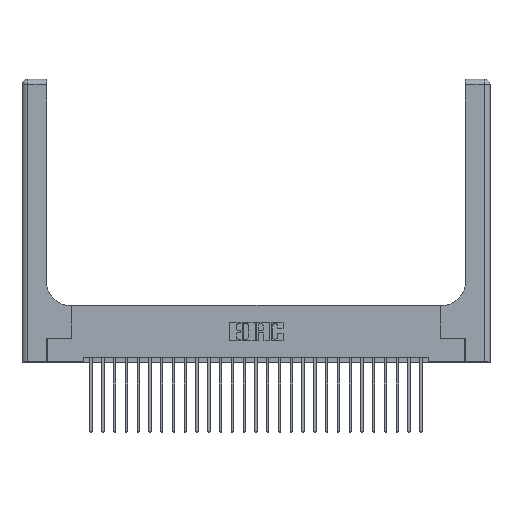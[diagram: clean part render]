
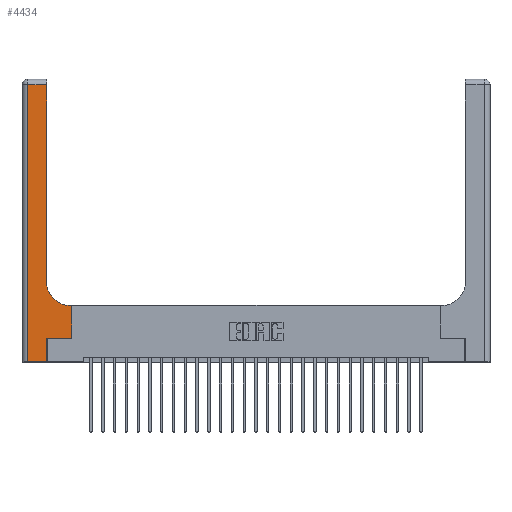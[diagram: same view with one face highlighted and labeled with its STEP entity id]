
A CAD part, top view. The second image highlights one B-rep face of the part: STEP entity #4434.
In plain terms, the highlighted planar face has unit normal (0, 0, 1).
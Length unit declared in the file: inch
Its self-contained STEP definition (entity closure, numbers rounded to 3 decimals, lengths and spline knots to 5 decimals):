
#78 = VERTEX_POINT ( 'NONE', #9043 ) ;
#508 = LINE ( 'NONE', #7594, #12063 ) ;
#548 = LINE ( 'NONE', #16430, #21140 ) ;
#1454 = CARTESIAN_POINT ( 'NONE',  ( 0.528, 0.25, 0.37 ) ) ;
#1733 = ORIENTED_EDGE ( 'NONE', *, *, #17524, .T. ) ;
#2019 = DIRECTION ( 'NONE',  ( -1., 0., 0. ) ) ;
#2164 = CARTESIAN_POINT ( 'NONE',  ( 0.26, 3., 0.37 ) ) ;
#2184 = DIRECTION ( 'NONE',  ( 0., 0., -1. ) ) ;
#2272 = AXIS2_PLACEMENT_3D ( 'NONE', #25510, #25422, #15429 ) ;
#2430 = CARTESIAN_POINT ( 'NONE',  ( 0.528, 0.6, 0.37 ) ) ;
#2673 = VERTEX_POINT ( 'NONE', #6800 ) ;
#2929 = DIRECTION ( 'NONE',  ( 1., 0., 0. ) ) ;
#3951 = DIRECTION ( 'NONE',  ( 0., 1., 0. ) ) ;
#4120 = CARTESIAN_POINT ( 'NONE',  ( 0., 3., 0.37 ) ) ;
#4323 = LINE ( 'NONE', #17794, #13982 ) ;
#4434 = ADVANCED_FACE ( 'NONE', ( #13801 ), #10124, .F. ) ;
#4783 = VERTEX_POINT ( 'NONE', #7234 ) ;
#5087 = CARTESIAN_POINT ( 'NONE',  ( 0.06, 2.94, 0.37 ) ) ;
#5290 = LINE ( 'NONE', #25007, #7183 ) ;
#6087 = CARTESIAN_POINT ( 'NONE',  ( 0.06, 0., 0.37 ) ) ;
#6323 = EDGE_CURVE ( 'NONE', #22401, #2673, #5290, .T. ) ;
#6440 = ORIENTED_EDGE ( 'NONE', *, *, #7628, .T. ) ;
#6583 = VERTEX_POINT ( 'NONE', #2430 ) ;
#6800 = CARTESIAN_POINT ( 'NONE',  ( 0.265, 0., 0.37 ) ) ;
#7183 = VECTOR ( 'NONE', #2929, 39.37008 ) ;
#7234 = CARTESIAN_POINT ( 'NONE',  ( 0.528, 0.25, 0.37 ) ) ;
#7251 = VERTEX_POINT ( 'NONE', #5087 ) ;
#7277 = EDGE_CURVE ( 'NONE', #19356, #11826, #9938, .T. ) ;
#7475 = CARTESIAN_POINT ( 'NONE',  ( 0.51, 0.6, 0.37 ) ) ;
#7594 = CARTESIAN_POINT ( 'NONE',  ( 0.26, 0.6, 0.37 ) ) ;
#7628 = EDGE_CURVE ( 'NONE', #7251, #22401, #548, .T. ) ;
#8007 = CARTESIAN_POINT ( 'NONE',  ( 0.26, 0.85, 0.37 ) ) ;
#8088 = DIRECTION ( 'NONE',  ( -1., 0., 0. ) ) ;
#9043 = CARTESIAN_POINT ( 'NONE',  ( 0.265, 0.25, 0.37 ) ) ;
#9224 = LINE ( 'NONE', #21959, #16116 ) ;
#9255 = EDGE_CURVE ( 'NONE', #6583, #19356, #508, .T. ) ;
#9912 = ORIENTED_EDGE ( 'NONE', *, *, #9255, .T. ) ;
#9938 = CIRCLE ( 'NONE', #2272, 0.25 ) ;
#10124 = PLANE ( 'NONE',  #14109 ) ;
#10501 = DIRECTION ( 'NONE',  ( 0., -1., 0. ) ) ;
#11153 = DIRECTION ( 'NONE',  ( 0., 1., 0. ) ) ;
#11826 = VERTEX_POINT ( 'NONE', #8007 ) ;
#11964 = LINE ( 'NONE', #25677, #25102 ) ;
#12063 = VECTOR ( 'NONE', #21534, 39.37008 ) ;
#13184 = VECTOR ( 'NONE', #15936, 39.37008 ) ;
#13801 = FACE_OUTER_BOUND ( 'NONE', #18793, .T. ) ;
#13982 = VECTOR ( 'NONE', #3951, 39.37008 ) ;
#14109 = AXIS2_PLACEMENT_3D ( 'NONE', #4120, #2184, #2019 ) ;
#14334 = EDGE_CURVE ( 'NONE', #2673, #78, #4323, .T. ) ;
#15190 = EDGE_CURVE ( 'NONE', #4783, #6583, #16409, .T. ) ;
#15260 = DIRECTION ( 'NONE',  ( 1., 0., 0. ) ) ;
#15352 = EDGE_CURVE ( 'NONE', #23142, #7251, #9224, .T. ) ;
#15429 = DIRECTION ( 'NONE',  ( 1., 0., 0. ) ) ;
#15767 = ORIENTED_EDGE ( 'NONE', *, *, #15352, .T. ) ;
#15936 = DIRECTION ( 'NONE',  ( 0., 1., 0. ) ) ;
#16116 = VECTOR ( 'NONE', #8088, 39.37008 ) ;
#16409 = LINE ( 'NONE', #1454, #25185 ) ;
#16430 = CARTESIAN_POINT ( 'NONE',  ( 0.06, 3., 0.37 ) ) ;
#16789 = ORIENTED_EDGE ( 'NONE', *, *, #15190, .T. ) ;
#17359 = ORIENTED_EDGE ( 'NONE', *, *, #23991, .T. ) ;
#17524 = EDGE_CURVE ( 'NONE', #11826, #23142, #24750, .T. ) ;
#17794 = CARTESIAN_POINT ( 'NONE',  ( 0.265, 0., 0.37 ) ) ;
#18410 = ORIENTED_EDGE ( 'NONE', *, *, #6323, .T. ) ;
#18793 = EDGE_LOOP ( 'NONE', ( #1733, #15767, #6440, #18410, #22979, #17359, #16789, #9912, #19726 ) ) ;
#19356 = VERTEX_POINT ( 'NONE', #7475 ) ;
#19726 = ORIENTED_EDGE ( 'NONE', *, *, #7277, .T. ) ;
#20324 = CARTESIAN_POINT ( 'NONE',  ( 0.26, 2.94, 0.37 ) ) ;
#21140 = VECTOR ( 'NONE', #10501, 39.37008 ) ;
#21534 = DIRECTION ( 'NONE',  ( -1., 0., 0. ) ) ;
#21959 = CARTESIAN_POINT ( 'NONE',  ( 0., 2.94, 0.37 ) ) ;
#22401 = VERTEX_POINT ( 'NONE', #6087 ) ;
#22979 = ORIENTED_EDGE ( 'NONE', *, *, #14334, .T. ) ;
#23142 = VERTEX_POINT ( 'NONE', #20324 ) ;
#23991 = EDGE_CURVE ( 'NONE', #78, #4783, #11964, .T. ) ;
#24750 = LINE ( 'NONE', #2164, #13184 ) ;
#25007 = CARTESIAN_POINT ( 'NONE',  ( 0., 0., 0.37 ) ) ;
#25102 = VECTOR ( 'NONE', #15260, 39.37008 ) ;
#25185 = VECTOR ( 'NONE', #11153, 39.37008 ) ;
#25422 = DIRECTION ( 'NONE',  ( 0., 0., -1. ) ) ;
#25510 = CARTESIAN_POINT ( 'NONE',  ( 0.51, 0.85, 0.37 ) ) ;
#25677 = CARTESIAN_POINT ( 'NONE',  ( 0.265, 0.25, 0.37 ) ) ;
